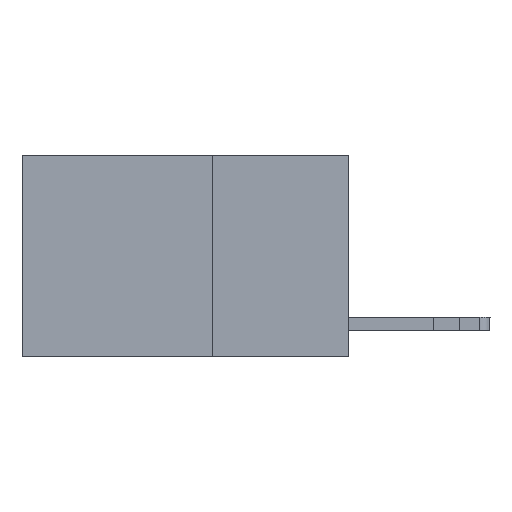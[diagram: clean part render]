
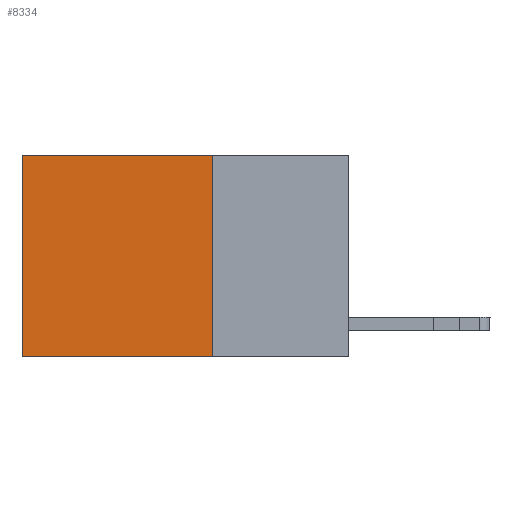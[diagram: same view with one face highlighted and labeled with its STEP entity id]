
A CAD part, left-side view. The second image highlights one B-rep face of the part: STEP entity #8334.
In plain terms, the highlighted planar face has unit normal (-1, 0, 0).
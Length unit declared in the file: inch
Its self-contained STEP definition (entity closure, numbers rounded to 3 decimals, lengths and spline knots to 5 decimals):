
#1164 = CARTESIAN_POINT ( 'NONE',  ( 0.2625, 0.25, -0.37 ) ) ;
#1206 = CARTESIAN_POINT ( 'NONE',  ( 0.2625, 0.25, 0. ) ) ;
#1239 = VECTOR ( 'NONE', #13812, 39.37008 ) ;
#1453 = LINE ( 'NONE', #9553, #1239 ) ;
#1540 = EDGE_CURVE ( 'NONE', #25187, #17665, #19358, .T. ) ;
#2560 = ORIENTED_EDGE ( 'NONE', *, *, #13847, .T. ) ;
#2594 = ORIENTED_EDGE ( 'NONE', *, *, #9130, .T. ) ;
#3050 = PLANE ( 'NONE',  #7720 ) ;
#4412 = DIRECTION ( 'NONE',  ( 0., 0., -1. ) ) ;
#4807 = EDGE_CURVE ( 'NONE', #13543, #25187, #1453, .T. ) ;
#6249 = CARTESIAN_POINT ( 'NONE',  ( 0.2625, 0.6, 0. ) ) ;
#7290 = DIRECTION ( 'NONE',  ( 0., 1., 0. ) ) ;
#7720 = AXIS2_PLACEMENT_3D ( 'NONE', #10054, #18172, #25332 ) ;
#8334 = ADVANCED_FACE ( 'NONE', ( #15128 ), #3050, .F. ) ;
#8665 = CARTESIAN_POINT ( 'NONE',  ( 0.2625, 0.25, -0.37 ) ) ;
#9130 = EDGE_CURVE ( 'NONE', #13543, #15504, #12916, .T. ) ;
#9553 = CARTESIAN_POINT ( 'NONE',  ( 0.2625, 0.25, 0. ) ) ;
#9988 = VECTOR ( 'NONE', #4412, 39.37008 ) ;
#10054 = CARTESIAN_POINT ( 'NONE',  ( 0.2625, 0.25, 0. ) ) ;
#12916 = LINE ( 'NONE', #20993, #16246 ) ;
#13146 = VECTOR ( 'NONE', #7290, 39.37008 ) ;
#13543 = VERTEX_POINT ( 'NONE', #1206 ) ;
#13812 = DIRECTION ( 'NONE',  ( 0., 0., -1. ) ) ;
#13847 = EDGE_CURVE ( 'NONE', #15504, #17665, #22586, .T. ) ;
#14671 = ORIENTED_EDGE ( 'NONE', *, *, #1540, .F. ) ;
#15128 = FACE_OUTER_BOUND ( 'NONE', #21826, .T. ) ;
#15504 = VERTEX_POINT ( 'NONE', #6249 ) ;
#15926 = ORIENTED_EDGE ( 'NONE', *, *, #4807, .F. ) ;
#16246 = VECTOR ( 'NONE', #19282, 39.37008 ) ;
#17665 = VERTEX_POINT ( 'NONE', #18739 ) ;
#18172 = DIRECTION ( 'NONE',  ( 1., 0., 0. ) ) ;
#18739 = CARTESIAN_POINT ( 'NONE',  ( 0.2625, 0.6, -0.37 ) ) ;
#19282 = DIRECTION ( 'NONE',  ( 0., 1., 0. ) ) ;
#19358 = LINE ( 'NONE', #1164, #13146 ) ;
#20591 = CARTESIAN_POINT ( 'NONE',  ( 0.2625, 0.6, 0. ) ) ;
#20993 = CARTESIAN_POINT ( 'NONE',  ( 0.2625, 0.25, 0. ) ) ;
#21826 = EDGE_LOOP ( 'NONE', ( #2560, #14671, #15926, #2594 ) ) ;
#22586 = LINE ( 'NONE', #20591, #9988 ) ;
#25187 = VERTEX_POINT ( 'NONE', #8665 ) ;
#25332 = DIRECTION ( 'NONE',  ( 0., 0., -1. ) ) ;
